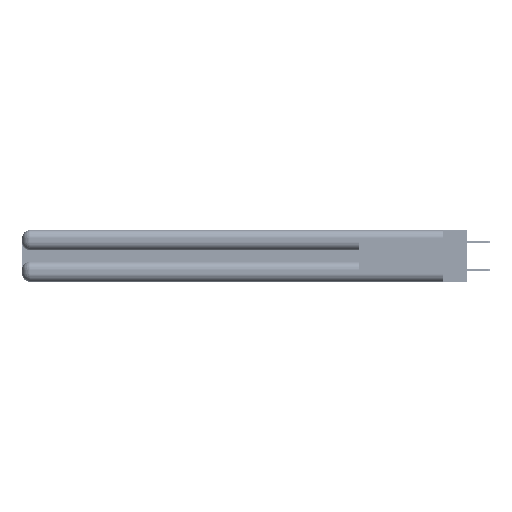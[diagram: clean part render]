
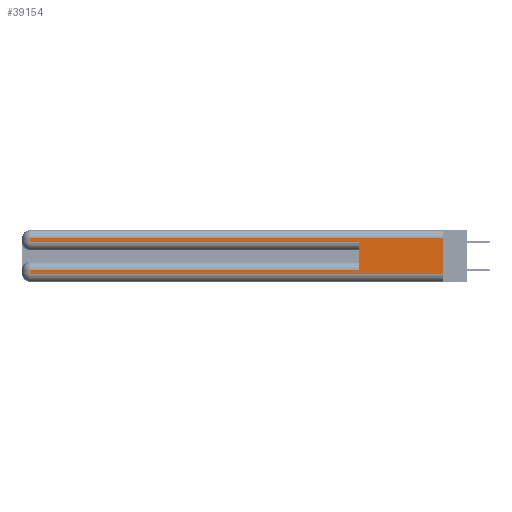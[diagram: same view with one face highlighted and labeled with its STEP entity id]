
A CAD part, left-side view. The second image highlights one B-rep face of the part: STEP entity #39154.
In plain terms, the highlighted planar face has unit normal (-1, 0, 0).
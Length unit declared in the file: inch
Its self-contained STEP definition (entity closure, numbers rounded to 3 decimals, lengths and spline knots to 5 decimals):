
#318 = CARTESIAN_POINT ( 'NONE',  ( 0., 0., 0.31 ) ) ;
#323 = LINE ( 'NONE', #10817, #46850 ) ;
#706 = VERTEX_POINT ( 'NONE', #36202 ) ;
#2022 = DIRECTION ( 'NONE',  ( 1., 0., 0. ) ) ;
#2657 = CARTESIAN_POINT ( 'NONE',  ( 0., 0., 0.31 ) ) ;
#2908 = ORIENTED_EDGE ( 'NONE', *, *, #52129, .T. ) ;
#3233 = VERTEX_POINT ( 'NONE', #28006 ) ;
#3509 = VERTEX_POINT ( 'NONE', #12518 ) ;
#3516 = CARTESIAN_POINT ( 'NONE',  ( 0., 0.6, 0.085 ) ) ;
#5762 = EDGE_CURVE ( 'NONE', #52496, #37602, #33781, .T. ) ;
#10062 = CARTESIAN_POINT ( 'NONE',  ( 0., 0., 0.06 ) ) ;
#10539 = VECTOR ( 'NONE', #28183, 39.37008 ) ;
#10547 = EDGE_CURVE ( 'NONE', #28426, #3233, #25613, .T. ) ;
#10817 = CARTESIAN_POINT ( 'NONE',  ( 0., 2.94, 0.37 ) ) ;
#11797 = CARTESIAN_POINT ( 'NONE',  ( 0., 0.6, 0.145 ) ) ;
#12153 = LINE ( 'NONE', #11797, #14897 ) ;
#12518 = CARTESIAN_POINT ( 'NONE',  ( 0., 2.94, 0.085 ) ) ;
#13764 = CARTESIAN_POINT ( 'NONE',  ( 0., 2.94, 0.285 ) ) ;
#14007 = VECTOR ( 'NONE', #42013, 39.37008 ) ;
#14063 = ORIENTED_EDGE ( 'NONE', *, *, #41974, .F. ) ;
#14897 = VECTOR ( 'NONE', #46663, 39.37008 ) ;
#14954 = DIRECTION ( 'NONE',  ( 0., 1., 0. ) ) ;
#15945 = AXIS2_PLACEMENT_3D ( 'NONE', #23846, #2022, #32652 ) ;
#16035 = EDGE_CURVE ( 'NONE', #52541, #706, #50310, .T. ) ;
#16607 = LINE ( 'NONE', #41885, #38420 ) ;
#18330 = ORIENTED_EDGE ( 'NONE', *, *, #5762, .T. ) ;
#18958 = VECTOR ( 'NONE', #27924, 39.37008 ) ;
#19167 = ORIENTED_EDGE ( 'NONE', *, *, #20441, .T. ) ;
#20441 = EDGE_CURVE ( 'NONE', #3233, #52496, #323, .T. ) ;
#23224 = DIRECTION ( 'NONE',  ( 0., -1., 0. ) ) ;
#23846 = CARTESIAN_POINT ( 'NONE',  ( 0., 0., 0.37 ) ) ;
#24450 = EDGE_LOOP ( 'NONE', ( #38852, #49668, #19167, #18330, #14063, #48453, #2908, #31062 ) ) ;
#24764 = EDGE_CURVE ( 'NONE', #45868, #3509, #48927, .T. ) ;
#25613 = LINE ( 'NONE', #2657, #14007 ) ;
#27103 = VECTOR ( 'NONE', #23224, 39.37008 ) ;
#27924 = DIRECTION ( 'NONE',  ( 0., 0., -1. ) ) ;
#28006 = CARTESIAN_POINT ( 'NONE',  ( 0., 2.94, 0.31 ) ) ;
#28111 = EDGE_CURVE ( 'NONE', #28426, #706, #16607, .T. ) ;
#28183 = DIRECTION ( 'NONE',  ( 0., -1., 0. ) ) ;
#28366 = CARTESIAN_POINT ( 'NONE',  ( 0., 0., 0.285 ) ) ;
#28426 = VERTEX_POINT ( 'NONE', #318 ) ;
#29535 = CARTESIAN_POINT ( 'NONE',  ( 0., 0.6, 0.285 ) ) ;
#31062 = ORIENTED_EDGE ( 'NONE', *, *, #16035, .T. ) ;
#32652 = DIRECTION ( 'NONE',  ( 0., 0., -1. ) ) ;
#33781 = LINE ( 'NONE', #28366, #10539 ) ;
#35993 = VECTOR ( 'NONE', #14954, 39.37008 ) ;
#36202 = CARTESIAN_POINT ( 'NONE',  ( 0., 0., 0.06 ) ) ;
#36887 = CARTESIAN_POINT ( 'NONE',  ( 0., 0., 0.085 ) ) ;
#37602 = VERTEX_POINT ( 'NONE', #29535 ) ;
#38420 = VECTOR ( 'NONE', #46252, 39.37008 ) ;
#38852 = ORIENTED_EDGE ( 'NONE', *, *, #28111, .F. ) ;
#39154 = ADVANCED_FACE ( 'NONE', ( #53847 ), #54313, .F. ) ;
#41885 = CARTESIAN_POINT ( 'NONE',  ( 0., 0., 0.37 ) ) ;
#41974 = EDGE_CURVE ( 'NONE', #45868, #37602, #12153, .T. ) ;
#42013 = DIRECTION ( 'NONE',  ( 0., 1., 0. ) ) ;
#45707 = DIRECTION ( 'NONE',  ( 0., 0., -1. ) ) ;
#45868 = VERTEX_POINT ( 'NONE', #3516 ) ;
#46252 = DIRECTION ( 'NONE',  ( 0., 0., -1. ) ) ;
#46663 = DIRECTION ( 'NONE',  ( 0., 0., 1. ) ) ;
#46850 = VECTOR ( 'NONE', #45707, 39.37008 ) ;
#48453 = ORIENTED_EDGE ( 'NONE', *, *, #24764, .T. ) ;
#48823 = CARTESIAN_POINT ( 'NONE',  ( 0., 2.94, 0.06 ) ) ;
#48927 = LINE ( 'NONE', #36887, #35993 ) ;
#49668 = ORIENTED_EDGE ( 'NONE', *, *, #10547, .T. ) ;
#50310 = LINE ( 'NONE', #10062, #27103 ) ;
#52129 = EDGE_CURVE ( 'NONE', #3509, #52541, #52331, .T. ) ;
#52331 = LINE ( 'NONE', #54008, #18958 ) ;
#52496 = VERTEX_POINT ( 'NONE', #13764 ) ;
#52541 = VERTEX_POINT ( 'NONE', #48823 ) ;
#53847 = FACE_OUTER_BOUND ( 'NONE', #24450, .T. ) ;
#54008 = CARTESIAN_POINT ( 'NONE',  ( 0., 2.94, 0.37 ) ) ;
#54313 = PLANE ( 'NONE',  #15945 ) ;
